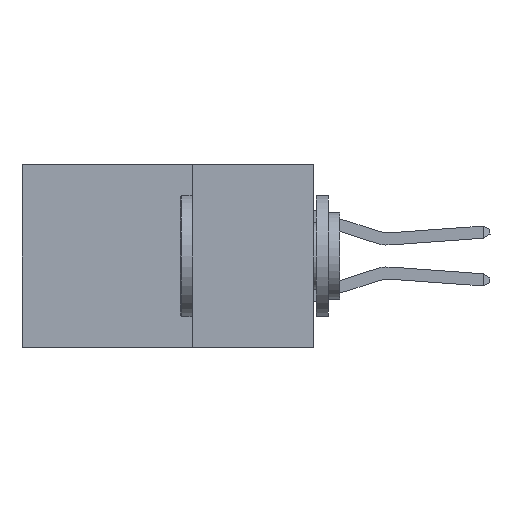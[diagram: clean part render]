
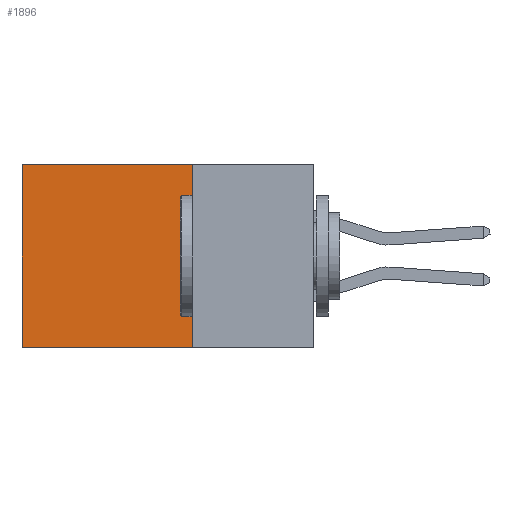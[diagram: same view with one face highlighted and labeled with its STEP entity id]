
A CAD part, left-side view. The second image highlights one B-rep face of the part: STEP entity #1896.
In plain terms, the highlighted planar face has unit normal (-1, 0, 0).
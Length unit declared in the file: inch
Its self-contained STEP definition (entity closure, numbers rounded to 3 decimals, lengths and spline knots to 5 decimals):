
#386 = DIRECTION ( 'NONE',  ( 1., 0., 0. ) ) ;
#421 = EDGE_LOOP ( 'NONE', ( #14214, #1667, #13298, #12699 ) ) ;
#1090 = CARTESIAN_POINT ( 'NONE',  ( 0.2875, 0.25, 0. ) ) ;
#1216 = CARTESIAN_POINT ( 'NONE',  ( 0.2875, 0.25, -0.375 ) ) ;
#1667 = ORIENTED_EDGE ( 'NONE', *, *, #12477, .F. ) ;
#1758 = VECTOR ( 'NONE', #14146, 39.37008 ) ;
#1896 = ADVANCED_FACE ( 'NONE', ( #5499 ), #7084, .F. ) ;
#2381 = VERTEX_POINT ( 'NONE', #3564 ) ;
#2461 = LINE ( 'NONE', #1216, #12365 ) ;
#2543 = EDGE_CURVE ( 'NONE', #2381, #4489, #12843, .T. ) ;
#2824 = LINE ( 'NONE', #5167, #1758 ) ;
#2896 = VECTOR ( 'NONE', #13143, 39.37008 ) ;
#2997 = EDGE_CURVE ( 'NONE', #4489, #9850, #2824, .T. ) ;
#3564 = CARTESIAN_POINT ( 'NONE',  ( 0.2875, 0.25, 0. ) ) ;
#3888 = DIRECTION ( 'NONE',  ( 0., 0., -1. ) ) ;
#4489 = VERTEX_POINT ( 'NONE', #12100 ) ;
#4508 = DIRECTION ( 'NONE',  ( 0., 1., 0. ) ) ;
#4774 = VECTOR ( 'NONE', #4508, 39.37008 ) ;
#5167 = CARTESIAN_POINT ( 'NONE',  ( 0.2875, 0.6, -0.375 ) ) ;
#5499 = FACE_OUTER_BOUND ( 'NONE', #421, .T. ) ;
#5741 = EDGE_CURVE ( 'NONE', #2381, #10628, #2461, .T. ) ;
#7084 = PLANE ( 'NONE',  #13151 ) ;
#8162 = CARTESIAN_POINT ( 'NONE',  ( 0.2875, 0.6, -0.375 ) ) ;
#8686 = CARTESIAN_POINT ( 'NONE',  ( 0.2875, 0.25, -0.375 ) ) ;
#9211 = CARTESIAN_POINT ( 'NONE',  ( 0.2875, 0.25, -0.375 ) ) ;
#9850 = VERTEX_POINT ( 'NONE', #8162 ) ;
#10628 = VERTEX_POINT ( 'NONE', #11994 ) ;
#10883 = LINE ( 'NONE', #8686, #2896 ) ;
#11430 = DIRECTION ( 'NONE',  ( 0., 0., -1. ) ) ;
#11994 = CARTESIAN_POINT ( 'NONE',  ( 0.2875, 0.25, -0.375 ) ) ;
#12100 = CARTESIAN_POINT ( 'NONE',  ( 0.2875, 0.6, 0. ) ) ;
#12365 = VECTOR ( 'NONE', #11430, 39.37008 ) ;
#12477 = EDGE_CURVE ( 'NONE', #10628, #9850, #10883, .T. ) ;
#12699 = ORIENTED_EDGE ( 'NONE', *, *, #2543, .T. ) ;
#12843 = LINE ( 'NONE', #1090, #4774 ) ;
#13143 = DIRECTION ( 'NONE',  ( 0., 1., 0. ) ) ;
#13151 = AXIS2_PLACEMENT_3D ( 'NONE', #9211, #386, #3888 ) ;
#13298 = ORIENTED_EDGE ( 'NONE', *, *, #5741, .F. ) ;
#14146 = DIRECTION ( 'NONE',  ( 0., 0., -1. ) ) ;
#14214 = ORIENTED_EDGE ( 'NONE', *, *, #2997, .T. ) ;
